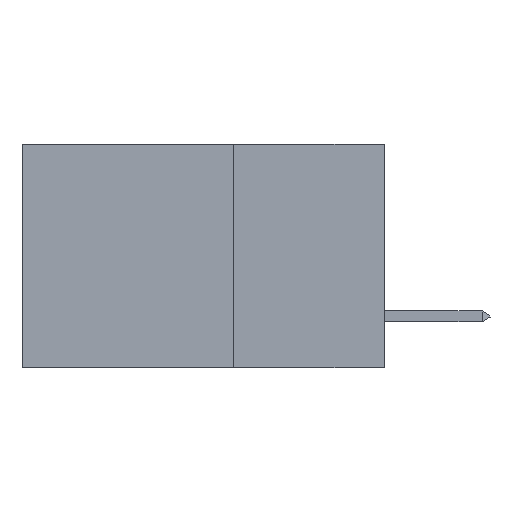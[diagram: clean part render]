
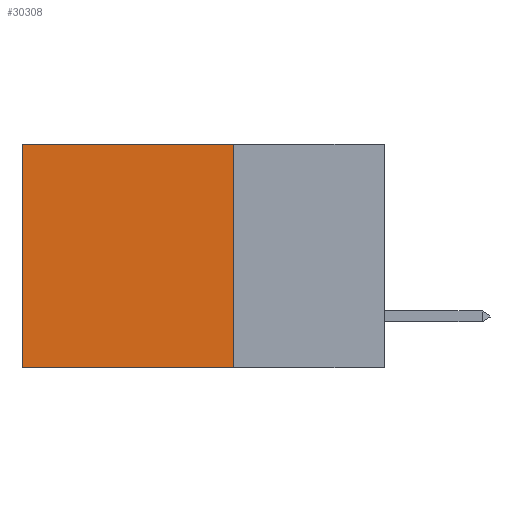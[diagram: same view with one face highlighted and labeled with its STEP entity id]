
A CAD part, left-side view. The second image highlights one B-rep face of the part: STEP entity #30308.
In plain terms, the highlighted planar face has unit normal (-1, 0, 0).
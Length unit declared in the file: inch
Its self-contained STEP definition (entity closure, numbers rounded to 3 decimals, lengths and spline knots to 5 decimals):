
#1719 = VERTEX_POINT ( 'NONE', #38253 ) ;
#2023 = VECTOR ( 'NONE', #24265, 39.37008 ) ;
#2257 = ORIENTED_EDGE ( 'NONE', *, *, #24443, .T. ) ;
#2741 = CARTESIAN_POINT ( 'NONE',  ( 0.2875, 0.25, 0. ) ) ;
#11556 = VECTOR ( 'NONE', #26690, 39.37008 ) ;
#12065 = CARTESIAN_POINT ( 'NONE',  ( 0.2875, 0.25, -0.37 ) ) ;
#15835 = AXIS2_PLACEMENT_3D ( 'NONE', #32765, #32458, #44168 ) ;
#24265 = DIRECTION ( 'NONE',  ( 0., 1., 0. ) ) ;
#24386 = VERTEX_POINT ( 'NONE', #27165 ) ;
#24443 = EDGE_CURVE ( 'NONE', #1719, #24386, #32673, .T. ) ;
#24539 = CARTESIAN_POINT ( 'NONE',  ( 0.2875, 0.25, 0. ) ) ;
#25362 = VECTOR ( 'NONE', #38205, 39.37008 ) ;
#26422 = EDGE_LOOP ( 'NONE', ( #2257, #27102, #29485, #42905 ) ) ;
#26690 = DIRECTION ( 'NONE',  ( 0., 0., -1. ) ) ;
#27102 = ORIENTED_EDGE ( 'NONE', *, *, #46482, .F. ) ;
#27165 = CARTESIAN_POINT ( 'NONE',  ( 0.2875, 0.6, -0.37 ) ) ;
#29485 = ORIENTED_EDGE ( 'NONE', *, *, #41128, .F. ) ;
#30307 = VECTOR ( 'NONE', #40198, 39.37008 ) ;
#30308 = ADVANCED_FACE ( 'NONE', ( #36500 ), #44013, .F. ) ;
#31427 = VERTEX_POINT ( 'NONE', #2741 ) ;
#32414 = LINE ( 'NONE', #12065, #25362 ) ;
#32458 = DIRECTION ( 'NONE',  ( 1., 0., 0. ) ) ;
#32673 = LINE ( 'NONE', #34522, #11556 ) ;
#32765 = CARTESIAN_POINT ( 'NONE',  ( 0.2875, 0.25, 0. ) ) ;
#33061 = VERTEX_POINT ( 'NONE', #46464 ) ;
#34226 = LINE ( 'NONE', #42562, #2023 ) ;
#34522 = CARTESIAN_POINT ( 'NONE',  ( 0.2875, 0.6, 0. ) ) ;
#36500 = FACE_OUTER_BOUND ( 'NONE', #26422, .T. ) ;
#38205 = DIRECTION ( 'NONE',  ( 0., 1., 0. ) ) ;
#38253 = CARTESIAN_POINT ( 'NONE',  ( 0.2875, 0.6, 0. ) ) ;
#40198 = DIRECTION ( 'NONE',  ( 0., 0., -1. ) ) ;
#40816 = LINE ( 'NONE', #24539, #30307 ) ;
#41128 = EDGE_CURVE ( 'NONE', #31427, #33061, #40816, .T. ) ;
#42562 = CARTESIAN_POINT ( 'NONE',  ( 0.2875, 0.25, 0. ) ) ;
#42689 = EDGE_CURVE ( 'NONE', #31427, #1719, #34226, .T. ) ;
#42905 = ORIENTED_EDGE ( 'NONE', *, *, #42689, .T. ) ;
#44013 = PLANE ( 'NONE',  #15835 ) ;
#44168 = DIRECTION ( 'NONE',  ( 0., 0., -1. ) ) ;
#46464 = CARTESIAN_POINT ( 'NONE',  ( 0.2875, 0.25, -0.37 ) ) ;
#46482 = EDGE_CURVE ( 'NONE', #33061, #24386, #32414, .T. ) ;
